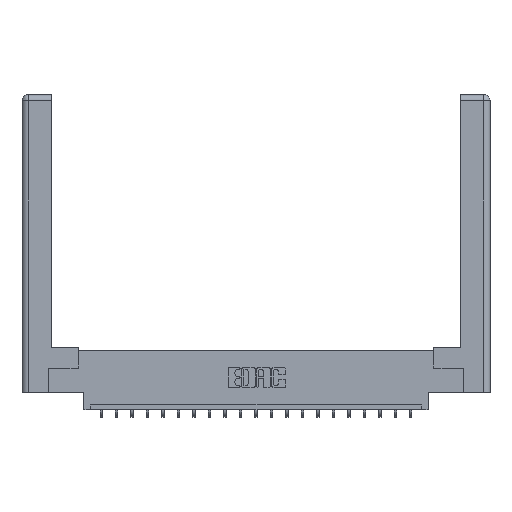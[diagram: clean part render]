
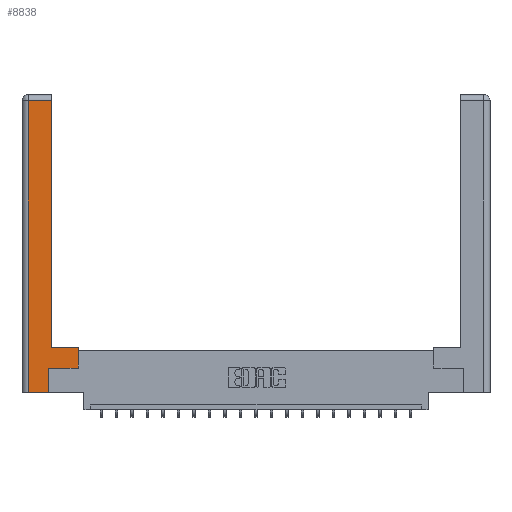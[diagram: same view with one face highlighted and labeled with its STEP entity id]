
A CAD part, top view. The second image highlights one B-rep face of the part: STEP entity #8838.
In plain terms, the highlighted planar face has unit normal (0, 0, 1).
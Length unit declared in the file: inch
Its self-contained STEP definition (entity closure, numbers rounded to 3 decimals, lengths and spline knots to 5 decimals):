
#486 = FACE_OUTER_BOUND ( 'NONE', #19628, .T. ) ;
#653 = EDGE_CURVE ( 'NONE', #17224, #12038, #15610, .T. ) ;
#1733 = CARTESIAN_POINT ( 'NONE',  ( 0.565, 0.245, 0. ) ) ;
#1760 = VECTOR ( 'NONE', #20227, 39.37008 ) ;
#2057 = VECTOR ( 'NONE', #7555, 39.37008 ) ;
#2078 = LINE ( 'NONE', #17773, #17647 ) ;
#2112 = ORIENTED_EDGE ( 'NONE', *, *, #11650, .T. ) ;
#2687 = DIRECTION ( 'NONE',  ( -1., 0., 0. ) ) ;
#3026 = ORIENTED_EDGE ( 'NONE', *, *, #18839, .T. ) ;
#3477 = ORIENTED_EDGE ( 'NONE', *, *, #20402, .T. ) ;
#4063 = VERTEX_POINT ( 'NONE', #16974 ) ;
#4086 = CARTESIAN_POINT ( 'NONE',  ( 0.265, 0., 0. ) ) ;
#4350 = VERTEX_POINT ( 'NONE', #1733 ) ;
#4383 = VERTEX_POINT ( 'NONE', #15067 ) ;
#4900 = EDGE_CURVE ( 'NONE', #4063, #4350, #12422, .T. ) ;
#5344 = ORIENTED_EDGE ( 'NONE', *, *, #14387, .T. ) ;
#6067 = LINE ( 'NONE', #16614, #1760 ) ;
#6676 = CARTESIAN_POINT ( 'NONE',  ( 0.295, 2.94, 0. ) ) ;
#7555 = DIRECTION ( 'NONE',  ( 0., 1., 0. ) ) ;
#7703 = CARTESIAN_POINT ( 'NONE',  ( 0.565, 0.45, 0. ) ) ;
#8708 = VERTEX_POINT ( 'NONE', #9785 ) ;
#8838 = ADVANCED_FACE ( 'NONE', ( #486 ), #14307, .F. ) ;
#8878 = CARTESIAN_POINT ( 'NONE',  ( 0.295, 0.45, 0. ) ) ;
#9096 = LINE ( 'NONE', #21103, #9867 ) ;
#9213 = VECTOR ( 'NONE', #19155, 39.37008 ) ;
#9361 = CARTESIAN_POINT ( 'NONE',  ( 0.295, 3., 0. ) ) ;
#9583 = CARTESIAN_POINT ( 'NONE',  ( 0., 0., 0. ) ) ;
#9785 = CARTESIAN_POINT ( 'NONE',  ( 0.565, 0.45, 0. ) ) ;
#9867 = VECTOR ( 'NONE', #11392, 39.37008 ) ;
#11057 = CARTESIAN_POINT ( 'NONE',  ( 0.265, 0.245, 0. ) ) ;
#11239 = DIRECTION ( 'NONE',  ( -1., 0., 0. ) ) ;
#11392 = DIRECTION ( 'NONE',  ( -1., 0., 0. ) ) ;
#11650 = EDGE_CURVE ( 'NONE', #4350, #8708, #17623, .T. ) ;
#12038 = VERTEX_POINT ( 'NONE', #6676 ) ;
#12306 = VERTEX_POINT ( 'NONE', #4086 ) ;
#12422 = LINE ( 'NONE', #15856, #16498 ) ;
#12534 = DIRECTION ( 'NONE',  ( 1., 0., 0. ) ) ;
#13118 = EDGE_CURVE ( 'NONE', #4383, #15502, #6067, .T. ) ;
#14307 = PLANE ( 'NONE',  #20773 ) ;
#14387 = EDGE_CURVE ( 'NONE', #12038, #4383, #9096, .T. ) ;
#14433 = DIRECTION ( 'NONE',  ( 1., 0., 0. ) ) ;
#14599 = VECTOR ( 'NONE', #20673, 39.37008 ) ;
#14706 = ORIENTED_EDGE ( 'NONE', *, *, #20695, .T. ) ;
#14829 = LINE ( 'NONE', #11057, #9213 ) ;
#15067 = CARTESIAN_POINT ( 'NONE',  ( 0.0615, 2.94, 0. ) ) ;
#15502 = VERTEX_POINT ( 'NONE', #16606 ) ;
#15610 = LINE ( 'NONE', #9361, #14599 ) ;
#15856 = CARTESIAN_POINT ( 'NONE',  ( 0.565, 0.245, 0. ) ) ;
#16210 = ORIENTED_EDGE ( 'NONE', *, *, #4900, .T. ) ;
#16498 = VECTOR ( 'NONE', #12534, 39.37008 ) ;
#16606 = CARTESIAN_POINT ( 'NONE',  ( 0.0615, 0., 0. ) ) ;
#16614 = CARTESIAN_POINT ( 'NONE',  ( 0.0615, 0., 0. ) ) ;
#16974 = CARTESIAN_POINT ( 'NONE',  ( 0.265, 0.245, 0. ) ) ;
#17224 = VERTEX_POINT ( 'NONE', #8878 ) ;
#17461 = LINE ( 'NONE', #19007, #20572 ) ;
#17623 = LINE ( 'NONE', #7703, #2057 ) ;
#17647 = VECTOR ( 'NONE', #14433, 39.37008 ) ;
#17773 = CARTESIAN_POINT ( 'NONE',  ( 0.265, 0., 0. ) ) ;
#17993 = ORIENTED_EDGE ( 'NONE', *, *, #13118, .T. ) ;
#18839 = EDGE_CURVE ( 'NONE', #8708, #17224, #17461, .T. ) ;
#18933 = ORIENTED_EDGE ( 'NONE', *, *, #653, .T. ) ;
#19007 = CARTESIAN_POINT ( 'NONE',  ( 0.295, 0.45, 0. ) ) ;
#19155 = DIRECTION ( 'NONE',  ( 0., 1., 0. ) ) ;
#19338 = DIRECTION ( 'NONE',  ( 0., 0., -1. ) ) ;
#19628 = EDGE_LOOP ( 'NONE', ( #18933, #5344, #17993, #3477, #14706, #16210, #2112, #3026 ) ) ;
#20227 = DIRECTION ( 'NONE',  ( 0., -1., 0. ) ) ;
#20402 = EDGE_CURVE ( 'NONE', #15502, #12306, #2078, .T. ) ;
#20572 = VECTOR ( 'NONE', #2687, 39.37008 ) ;
#20673 = DIRECTION ( 'NONE',  ( 0., 1., 0. ) ) ;
#20695 = EDGE_CURVE ( 'NONE', #12306, #4063, #14829, .T. ) ;
#20773 = AXIS2_PLACEMENT_3D ( 'NONE', #9583, #19338, #11239 ) ;
#21103 = CARTESIAN_POINT ( 'NONE',  ( 0.0615, 2.94, 0. ) ) ;
